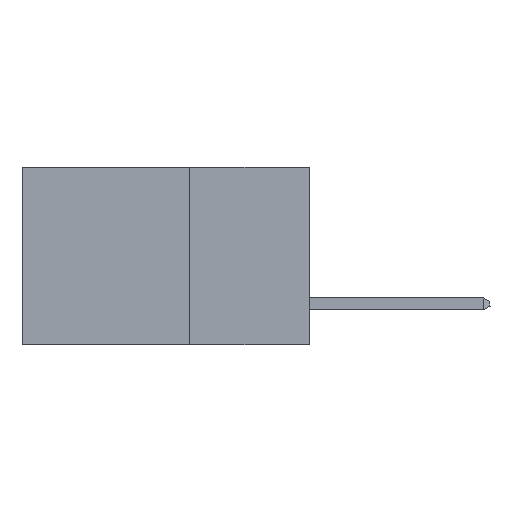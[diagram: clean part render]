
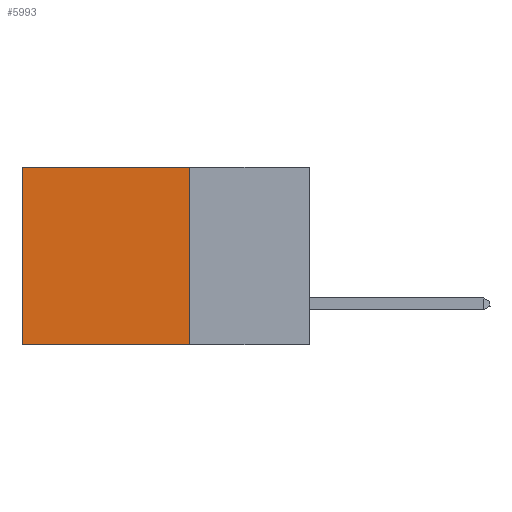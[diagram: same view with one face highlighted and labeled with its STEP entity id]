
A CAD part, left-side view. The second image highlights one B-rep face of the part: STEP entity #5993.
In plain terms, the highlighted planar face has unit normal (-1, 0, 0).
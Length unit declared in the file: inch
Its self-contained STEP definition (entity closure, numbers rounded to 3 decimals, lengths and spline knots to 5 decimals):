
#1502 = CARTESIAN_POINT ( 'NONE',  ( 0.2875, 0.6, -0.37 ) ) ;
#1639 = CARTESIAN_POINT ( 'NONE',  ( 0.2875, 0.6, 0. ) ) ;
#2882 = FACE_OUTER_BOUND ( 'NONE', #5086, .T. ) ;
#2914 = ORIENTED_EDGE ( 'NONE', *, *, #15323, .F. ) ;
#3462 = LINE ( 'NONE', #8348, #4622 ) ;
#4622 = VECTOR ( 'NONE', #16758, 39.37008 ) ;
#5086 = EDGE_LOOP ( 'NONE', ( #15697, #2914, #6791, #17760 ) ) ;
#5199 = CARTESIAN_POINT ( 'NONE',  ( 0.2875, 0.25, 0. ) ) ;
#5434 = CARTESIAN_POINT ( 'NONE',  ( 0.2875, 0.25, -0.37 ) ) ;
#5993 = ADVANCED_FACE ( 'NONE', ( #2882 ), #17617, .F. ) ;
#6657 = DIRECTION ( 'NONE',  ( 0., 1., 0. ) ) ;
#6775 = VECTOR ( 'NONE', #6657, 39.37008 ) ;
#6791 = ORIENTED_EDGE ( 'NONE', *, *, #12422, .F. ) ;
#7288 = VECTOR ( 'NONE', #16700, 39.37008 ) ;
#7833 = EDGE_CURVE ( 'NONE', #15737, #16142, #20192, .T. ) ;
#8236 = LINE ( 'NONE', #5199, #20090 ) ;
#8348 = CARTESIAN_POINT ( 'NONE',  ( 0.2875, 0.25, 0. ) ) ;
#9934 = LINE ( 'NONE', #18666, #6775 ) ;
#11434 = CARTESIAN_POINT ( 'NONE',  ( 0.2875, 0.25, 0. ) ) ;
#12422 = EDGE_CURVE ( 'NONE', #18378, #18697, #3462, .T. ) ;
#13265 = DIRECTION ( 'NONE',  ( 0., 1., 0. ) ) ;
#14319 = CARTESIAN_POINT ( 'NONE',  ( 0.2875, 0.25, 0. ) ) ;
#15047 = CARTESIAN_POINT ( 'NONE',  ( 0.2875, 0.6, 0. ) ) ;
#15230 = AXIS2_PLACEMENT_3D ( 'NONE', #14319, #21320, #17728 ) ;
#15323 = EDGE_CURVE ( 'NONE', #18697, #16142, #9934, .T. ) ;
#15697 = ORIENTED_EDGE ( 'NONE', *, *, #7833, .T. ) ;
#15737 = VERTEX_POINT ( 'NONE', #1639 ) ;
#16142 = VERTEX_POINT ( 'NONE', #1502 ) ;
#16700 = DIRECTION ( 'NONE',  ( 0., 0., -1. ) ) ;
#16758 = DIRECTION ( 'NONE',  ( 0., 0., -1. ) ) ;
#17617 = PLANE ( 'NONE',  #15230 ) ;
#17728 = DIRECTION ( 'NONE',  ( 0., 0., -1. ) ) ;
#17760 = ORIENTED_EDGE ( 'NONE', *, *, #20174, .T. ) ;
#18378 = VERTEX_POINT ( 'NONE', #11434 ) ;
#18666 = CARTESIAN_POINT ( 'NONE',  ( 0.2875, 0.25, -0.37 ) ) ;
#18697 = VERTEX_POINT ( 'NONE', #5434 ) ;
#20090 = VECTOR ( 'NONE', #13265, 39.37008 ) ;
#20174 = EDGE_CURVE ( 'NONE', #18378, #15737, #8236, .T. ) ;
#20192 = LINE ( 'NONE', #15047, #7288 ) ;
#21320 = DIRECTION ( 'NONE',  ( 1., 0., 0. ) ) ;
